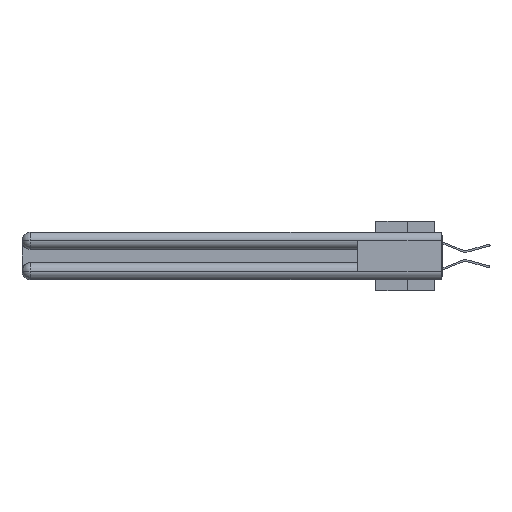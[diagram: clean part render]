
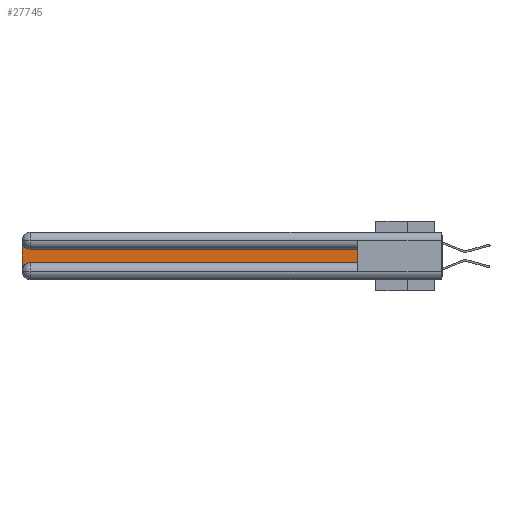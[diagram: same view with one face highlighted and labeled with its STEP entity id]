
A CAD part, left-side view. The second image highlights one B-rep face of the part: STEP entity #27745.
In plain terms, the highlighted planar face has unit normal (-1, 0, 0).
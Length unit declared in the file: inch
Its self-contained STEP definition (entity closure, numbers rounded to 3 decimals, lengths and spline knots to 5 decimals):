
#47 = ORIENTED_EDGE ( 'NONE', *, *, #7858, .T. ) ;
#484 = EDGE_CURVE ( 'NONE', #15048, #28451, #19578, .T. ) ;
#581 = VECTOR ( 'NONE', #30011, 39.37008 ) ;
#1170 = CARTESIAN_POINT ( 'NONE',  ( 0.075, 0.6, -0.2175 ) ) ;
#1377 = VERTEX_POINT ( 'NONE', #27679 ) ;
#1712 = CARTESIAN_POINT ( 'NONE',  ( 0.075, 3., -0.2775 ) ) ;
#1822 = DIRECTION ( 'NONE',  ( 0., 0., -1. ) ) ;
#2278 = CIRCLE ( 'NONE', #15141, 0.06 ) ;
#2695 = DIRECTION ( 'NONE',  ( 1., 0., 0. ) ) ;
#3660 = AXIS2_PLACEMENT_3D ( 'NONE', #10624, #2695, #5224 ) ;
#4304 = LINE ( 'NONE', #19759, #581 ) ;
#4530 = CARTESIAN_POINT ( 'NONE',  ( 0.075, 2.94, -0.2175 ) ) ;
#5100 = DIRECTION ( 'NONE',  ( 1., 0., 0. ) ) ;
#5144 = ORIENTED_EDGE ( 'NONE', *, *, #23936, .T. ) ;
#5224 = DIRECTION ( 'NONE',  ( 0., 0., -1. ) ) ;
#6096 = LINE ( 'NONE', #1170, #9656 ) ;
#7858 = EDGE_CURVE ( 'NONE', #25069, #22495, #4304, .T. ) ;
#8536 = VERTEX_POINT ( 'NONE', #4530 ) ;
#9069 = DIRECTION ( 'NONE',  ( 0., 1., 0. ) ) ;
#9234 = PLANE ( 'NONE',  #22862 ) ;
#9356 = CARTESIAN_POINT ( 'NONE',  ( 0.075, 0.6, -0.2175 ) ) ;
#9656 = VECTOR ( 'NONE', #16454, 39.37008 ) ;
#10624 = CARTESIAN_POINT ( 'NONE',  ( 0.075, 2.94, -0.2775 ) ) ;
#10818 = DIRECTION ( 'NONE',  ( 0., 0., -1. ) ) ;
#14255 = ORIENTED_EDGE ( 'NONE', *, *, #22818, .T. ) ;
#14523 = DIRECTION ( 'NONE',  ( 0., 0., 1. ) ) ;
#15048 = VERTEX_POINT ( 'NONE', #21642 ) ;
#15141 = AXIS2_PLACEMENT_3D ( 'NONE', #28267, #5100, #10818 ) ;
#16454 = DIRECTION ( 'NONE',  ( 0., -1., 0. ) ) ;
#17506 = CIRCLE ( 'NONE', #3660, 0.06 ) ;
#19578 = LINE ( 'NONE', #9356, #24352 ) ;
#19759 = CARTESIAN_POINT ( 'NONE',  ( 0.075, 3., -0.2175 ) ) ;
#21642 = CARTESIAN_POINT ( 'NONE',  ( 0.075, 0.6, -0.2175 ) ) ;
#22495 = VERTEX_POINT ( 'NONE', #1712 ) ;
#22818 = EDGE_CURVE ( 'NONE', #28451, #1377, #32235, .T. ) ;
#22862 = AXIS2_PLACEMENT_3D ( 'NONE', #29534, #32079, #1822 ) ;
#23936 = EDGE_CURVE ( 'NONE', #1377, #25069, #2278, .T. ) ;
#23967 = EDGE_LOOP ( 'NONE', ( #14255, #5144, #47, #32972, #33084, #29427 ) ) ;
#24352 = VECTOR ( 'NONE', #14523, 39.37008 ) ;
#24813 = VECTOR ( 'NONE', #9069, 39.37008 ) ;
#25069 = VERTEX_POINT ( 'NONE', #27939 ) ;
#27338 = CARTESIAN_POINT ( 'NONE',  ( 0.075, 0.6, -0.1225 ) ) ;
#27679 = CARTESIAN_POINT ( 'NONE',  ( 0.075, 2.94, -0.1225 ) ) ;
#27745 = ADVANCED_FACE ( 'NONE', ( #30048 ), #9234, .F. ) ;
#27939 = CARTESIAN_POINT ( 'NONE',  ( 0.075, 3., -0.0625 ) ) ;
#28267 = CARTESIAN_POINT ( 'NONE',  ( 0.075, 2.94, -0.0625 ) ) ;
#28451 = VERTEX_POINT ( 'NONE', #33204 ) ;
#29427 = ORIENTED_EDGE ( 'NONE', *, *, #484, .T. ) ;
#29464 = EDGE_CURVE ( 'NONE', #22495, #8536, #17506, .T. ) ;
#29534 = CARTESIAN_POINT ( 'NONE',  ( 0.075, 3., -0.1225 ) ) ;
#30011 = DIRECTION ( 'NONE',  ( 0., 0., -1. ) ) ;
#30048 = FACE_OUTER_BOUND ( 'NONE', #23967, .T. ) ;
#32079 = DIRECTION ( 'NONE',  ( 1., 0., 0. ) ) ;
#32235 = LINE ( 'NONE', #27338, #24813 ) ;
#32972 = ORIENTED_EDGE ( 'NONE', *, *, #29464, .T. ) ;
#33000 = EDGE_CURVE ( 'NONE', #8536, #15048, #6096, .T. ) ;
#33084 = ORIENTED_EDGE ( 'NONE', *, *, #33000, .T. ) ;
#33204 = CARTESIAN_POINT ( 'NONE',  ( 0.075, 0.6, -0.1225 ) ) ;
